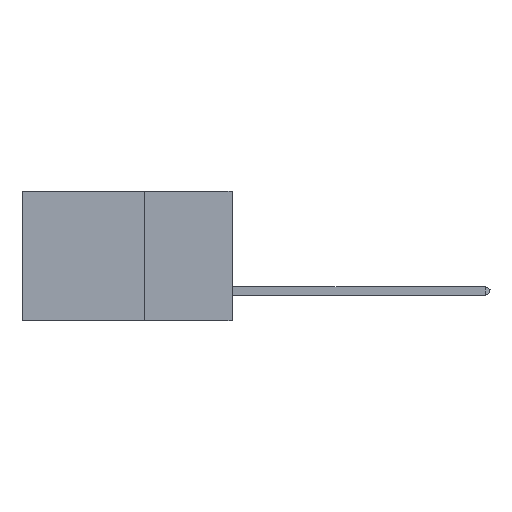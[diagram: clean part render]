
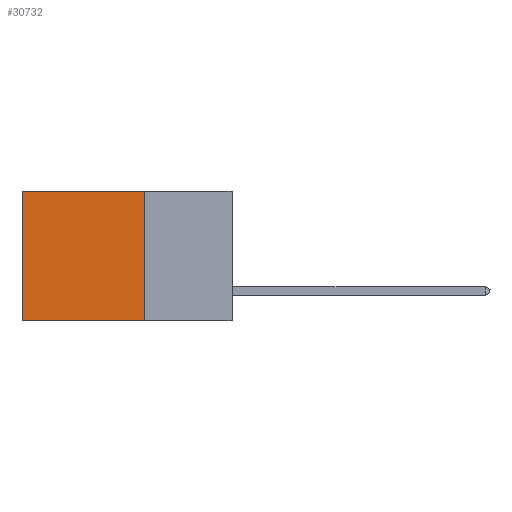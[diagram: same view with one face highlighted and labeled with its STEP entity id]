
A CAD part, left-side view. The second image highlights one B-rep face of the part: STEP entity #30732.
In plain terms, the highlighted planar face has unit normal (-1, 0, 0).
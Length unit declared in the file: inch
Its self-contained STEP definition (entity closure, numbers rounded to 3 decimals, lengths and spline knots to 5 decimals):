
#458 = VERTEX_POINT ( 'NONE', #30930 ) ;
#667 = VECTOR ( 'NONE', #949, 39.37008 ) ;
#949 = DIRECTION ( 'NONE',  ( 0., 1., 0. ) ) ;
#1484 = VECTOR ( 'NONE', #24676, 39.37008 ) ;
#2683 = ORIENTED_EDGE ( 'NONE', *, *, #9020, .F. ) ;
#4357 = CARTESIAN_POINT ( 'NONE',  ( 0.2875, 0.25, 0. ) ) ;
#6599 = AXIS2_PLACEMENT_3D ( 'NONE', #29141, #35824, #15914 ) ;
#9020 = EDGE_CURVE ( 'NONE', #15412, #458, #41270, .T. ) ;
#10377 = LINE ( 'NONE', #20693, #28080 ) ;
#11862 = CARTESIAN_POINT ( 'NONE',  ( 0.2875, 0.25, 0. ) ) ;
#11992 = CARTESIAN_POINT ( 'NONE',  ( 0.2875, 0.25, 0. ) ) ;
#12697 = ORIENTED_EDGE ( 'NONE', *, *, #24179, .T. ) ;
#13827 = CARTESIAN_POINT ( 'NONE',  ( 0.2875, 0.25, -0.37 ) ) ;
#14580 = ORIENTED_EDGE ( 'NONE', *, *, #34140, .F. ) ;
#15329 = PLANE ( 'NONE',  #6599 ) ;
#15412 = VERTEX_POINT ( 'NONE', #13827 ) ;
#15914 = DIRECTION ( 'NONE',  ( 0., 0., -1. ) ) ;
#19151 = VECTOR ( 'NONE', #37911, 39.37008 ) ;
#20158 = CARTESIAN_POINT ( 'NONE',  ( 0.2875, 0.6, 0. ) ) ;
#20693 = CARTESIAN_POINT ( 'NONE',  ( 0.2875, 0.6, 0. ) ) ;
#24179 = EDGE_CURVE ( 'NONE', #37052, #458, #10377, .T. ) ;
#24676 = DIRECTION ( 'NONE',  ( 0., 1., 0. ) ) ;
#26416 = LINE ( 'NONE', #11992, #1484 ) ;
#27226 = CARTESIAN_POINT ( 'NONE',  ( 0.2875, 0.25, -0.37 ) ) ;
#28080 = VECTOR ( 'NONE', #33778, 39.37008 ) ;
#28110 = EDGE_LOOP ( 'NONE', ( #12697, #2683, #14580, #31252 ) ) ;
#29141 = CARTESIAN_POINT ( 'NONE',  ( 0.2875, 0.25, 0. ) ) ;
#29551 = LINE ( 'NONE', #4357, #19151 ) ;
#30732 = ADVANCED_FACE ( 'NONE', ( #35222 ), #15329, .F. ) ;
#30930 = CARTESIAN_POINT ( 'NONE',  ( 0.2875, 0.6, -0.37 ) ) ;
#31252 = ORIENTED_EDGE ( 'NONE', *, *, #34248, .T. ) ;
#33778 = DIRECTION ( 'NONE',  ( 0., 0., -1. ) ) ;
#34140 = EDGE_CURVE ( 'NONE', #42381, #15412, #29551, .T. ) ;
#34248 = EDGE_CURVE ( 'NONE', #42381, #37052, #26416, .T. ) ;
#35222 = FACE_OUTER_BOUND ( 'NONE', #28110, .T. ) ;
#35824 = DIRECTION ( 'NONE',  ( 1., 0., 0. ) ) ;
#37052 = VERTEX_POINT ( 'NONE', #20158 ) ;
#37911 = DIRECTION ( 'NONE',  ( 0., 0., -1. ) ) ;
#41270 = LINE ( 'NONE', #27226, #667 ) ;
#42381 = VERTEX_POINT ( 'NONE', #11862 ) ;
